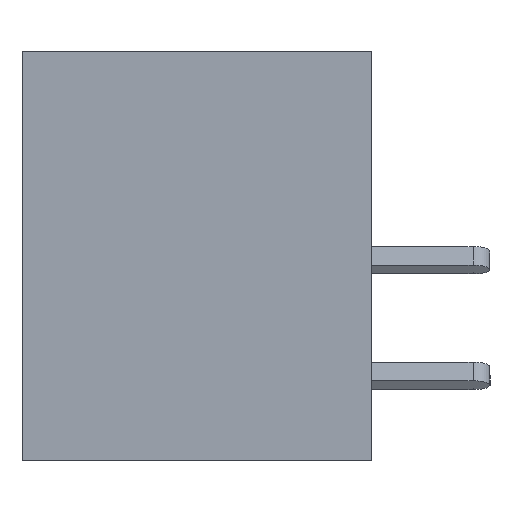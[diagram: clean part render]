
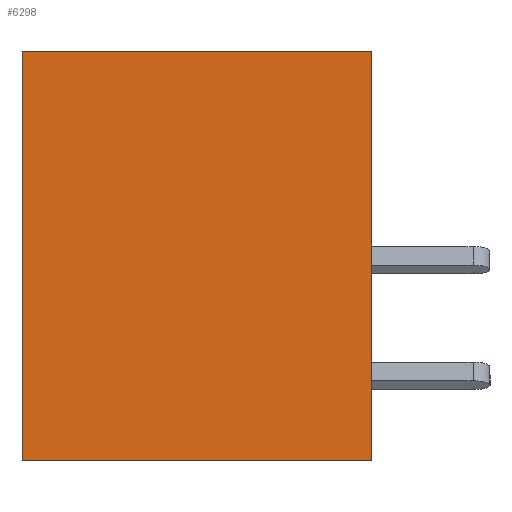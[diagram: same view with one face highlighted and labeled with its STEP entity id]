
A CAD part, left-side view. The second image highlights one B-rep face of the part: STEP entity #6298.
In plain terms, the highlighted planar face has unit normal (-1, 0, 0).
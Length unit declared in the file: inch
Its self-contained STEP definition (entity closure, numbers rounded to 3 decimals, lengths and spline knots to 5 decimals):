
#417 = LINE ( 'NONE', #12639, #8475 ) ;
#809 = VERTEX_POINT ( 'NONE', #9521 ) ;
#952 = EDGE_LOOP ( 'NONE', ( #3649, #13621, #12153, #3512 ) ) ;
#1718 = DIRECTION ( 'NONE',  ( 1., 0., 0. ) ) ;
#3512 = ORIENTED_EDGE ( 'NONE', *, *, #12346, .T. ) ;
#3649 = ORIENTED_EDGE ( 'NONE', *, *, #13110, .T. ) ;
#4278 = CARTESIAN_POINT ( 'NONE',  ( 0., 0.453, 0. ) ) ;
#4838 = FACE_OUTER_BOUND ( 'NONE', #952, .T. ) ;
#5134 = LINE ( 'NONE', #9376, #16231 ) ;
#5626 = VERTEX_POINT ( 'NONE', #8506 ) ;
#6298 = ADVANCED_FACE ( 'NONE', ( #4838 ), #8293, .F. ) ;
#6771 = DIRECTION ( 'NONE',  ( 0., -1., 0. ) ) ;
#7227 = CARTESIAN_POINT ( 'NONE',  ( 0., 0.453, -0.531 ) ) ;
#7279 = DIRECTION ( 'NONE',  ( 0., -1., 0. ) ) ;
#7426 = EDGE_CURVE ( 'NONE', #11635, #5626, #8088, .T. ) ;
#8023 = DIRECTION ( 'NONE',  ( 0., 0., 1. ) ) ;
#8088 = LINE ( 'NONE', #4278, #13600 ) ;
#8228 = CARTESIAN_POINT ( 'NONE',  ( 0., 0.453, 0. ) ) ;
#8293 = PLANE ( 'NONE',  #16139 ) ;
#8475 = VECTOR ( 'NONE', #11383, 39.37008 ) ;
#8506 = CARTESIAN_POINT ( 'NONE',  ( 0., 0.453, 0. ) ) ;
#9376 = CARTESIAN_POINT ( 'NONE',  ( 0., 0.453, 0. ) ) ;
#9521 = CARTESIAN_POINT ( 'NONE',  ( 0., 0., 0. ) ) ;
#9920 = VECTOR ( 'NONE', #7279, 39.37008 ) ;
#11233 = VERTEX_POINT ( 'NONE', #12472 ) ;
#11383 = DIRECTION ( 'NONE',  ( 0., 0., 1. ) ) ;
#11635 = VERTEX_POINT ( 'NONE', #14609 ) ;
#12153 = ORIENTED_EDGE ( 'NONE', *, *, #7426, .F. ) ;
#12297 = DIRECTION ( 'NONE',  ( 0., 0., -1. ) ) ;
#12346 = EDGE_CURVE ( 'NONE', #11635, #11233, #16021, .T. ) ;
#12472 = CARTESIAN_POINT ( 'NONE',  ( 0., 0., -0.531 ) ) ;
#12639 = CARTESIAN_POINT ( 'NONE',  ( 0., 0., 0. ) ) ;
#13110 = EDGE_CURVE ( 'NONE', #11233, #809, #417, .T. ) ;
#13348 = EDGE_CURVE ( 'NONE', #5626, #809, #5134, .T. ) ;
#13600 = VECTOR ( 'NONE', #8023, 39.37008 ) ;
#13621 = ORIENTED_EDGE ( 'NONE', *, *, #13348, .F. ) ;
#14609 = CARTESIAN_POINT ( 'NONE',  ( 0., 0.453, -0.531 ) ) ;
#16021 = LINE ( 'NONE', #7227, #9920 ) ;
#16139 = AXIS2_PLACEMENT_3D ( 'NONE', #8228, #1718, #12297 ) ;
#16231 = VECTOR ( 'NONE', #6771, 39.37008 ) ;
